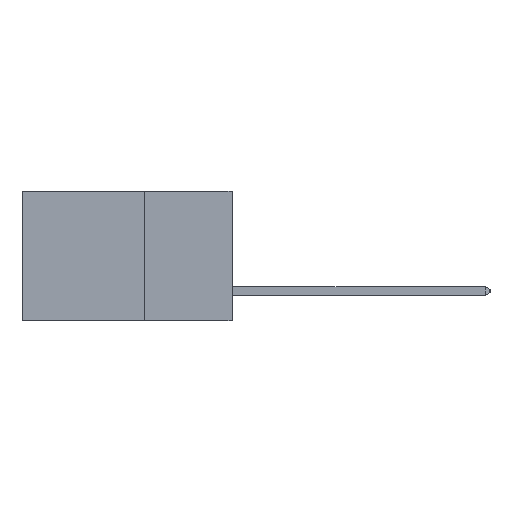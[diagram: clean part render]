
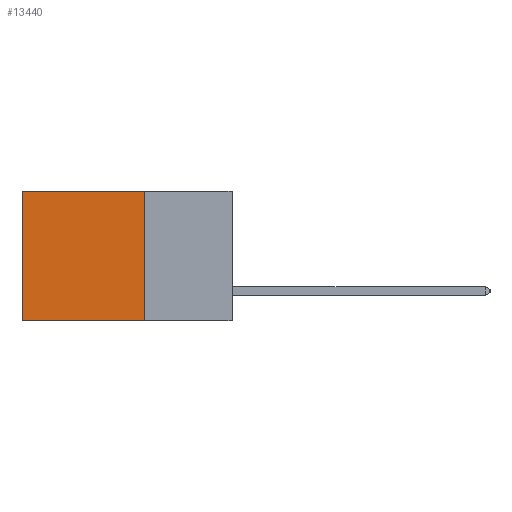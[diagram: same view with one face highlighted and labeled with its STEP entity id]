
A CAD part, left-side view. The second image highlights one B-rep face of the part: STEP entity #13440.
In plain terms, the highlighted planar face has unit normal (-1, 0, 0).
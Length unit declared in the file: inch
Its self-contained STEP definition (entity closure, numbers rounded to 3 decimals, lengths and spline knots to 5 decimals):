
#778 = DIRECTION ( 'NONE',  ( 0., 1., 0. ) ) ;
#859 = CARTESIAN_POINT ( 'NONE',  ( 0.2875, 0.6, 0. ) ) ;
#910 = VERTEX_POINT ( 'NONE', #22049 ) ;
#1428 = EDGE_CURVE ( 'NONE', #910, #34436, #5366, .T. ) ;
#1445 = CARTESIAN_POINT ( 'NONE',  ( 0.2875, 0.25, -0.37 ) ) ;
#2092 = VECTOR ( 'NONE', #778, 39.37008 ) ;
#3345 = ORIENTED_EDGE ( 'NONE', *, *, #1428, .F. ) ;
#3606 = ORIENTED_EDGE ( 'NONE', *, *, #17411, .T. ) ;
#3996 = CARTESIAN_POINT ( 'NONE',  ( 0.2875, 0.6, 0. ) ) ;
#4404 = FACE_OUTER_BOUND ( 'NONE', #30580, .T. ) ;
#5366 = LINE ( 'NONE', #29850, #17729 ) ;
#5537 = PLANE ( 'NONE',  #29040 ) ;
#9351 = CARTESIAN_POINT ( 'NONE',  ( 0.2875, 0.25, 0. ) ) ;
#10233 = DIRECTION ( 'NONE',  ( 0., 1., 0. ) ) ;
#11309 = VECTOR ( 'NONE', #10233, 39.37008 ) ;
#13084 = VERTEX_POINT ( 'NONE', #3996 ) ;
#13440 = ADVANCED_FACE ( 'NONE', ( #4404 ), #5537, .F. ) ;
#14177 = DIRECTION ( 'NONE',  ( 0., 0., -1. ) ) ;
#15941 = CARTESIAN_POINT ( 'NONE',  ( 0.2875, 0.25, -0.37 ) ) ;
#16196 = VECTOR ( 'NONE', #23536, 39.37008 ) ;
#17411 = EDGE_CURVE ( 'NONE', #13084, #27311, #23532, .T. ) ;
#17729 = VECTOR ( 'NONE', #23299, 39.37008 ) ;
#17967 = ORIENTED_EDGE ( 'NONE', *, *, #18187, .F. ) ;
#18119 = LINE ( 'NONE', #9351, #2092 ) ;
#18187 = EDGE_CURVE ( 'NONE', #34436, #27311, #18696, .T. ) ;
#18696 = LINE ( 'NONE', #1445, #11309 ) ;
#21540 = ORIENTED_EDGE ( 'NONE', *, *, #24482, .T. ) ;
#22049 = CARTESIAN_POINT ( 'NONE',  ( 0.2875, 0.25, 0. ) ) ;
#22135 = CARTESIAN_POINT ( 'NONE',  ( 0.2875, 0.6, -0.37 ) ) ;
#23299 = DIRECTION ( 'NONE',  ( 0., 0., -1. ) ) ;
#23532 = LINE ( 'NONE', #859, #16196 ) ;
#23536 = DIRECTION ( 'NONE',  ( 0., 0., -1. ) ) ;
#24482 = EDGE_CURVE ( 'NONE', #910, #13084, #18119, .T. ) ;
#25164 = CARTESIAN_POINT ( 'NONE',  ( 0.2875, 0.25, 0. ) ) ;
#27311 = VERTEX_POINT ( 'NONE', #22135 ) ;
#29040 = AXIS2_PLACEMENT_3D ( 'NONE', #25164, #30752, #14177 ) ;
#29850 = CARTESIAN_POINT ( 'NONE',  ( 0.2875, 0.25, 0. ) ) ;
#30580 = EDGE_LOOP ( 'NONE', ( #3606, #17967, #3345, #21540 ) ) ;
#30752 = DIRECTION ( 'NONE',  ( 1., 0., 0. ) ) ;
#34436 = VERTEX_POINT ( 'NONE', #15941 ) ;
